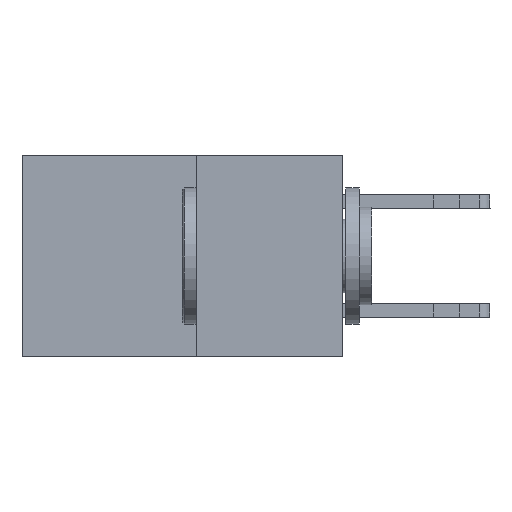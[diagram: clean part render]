
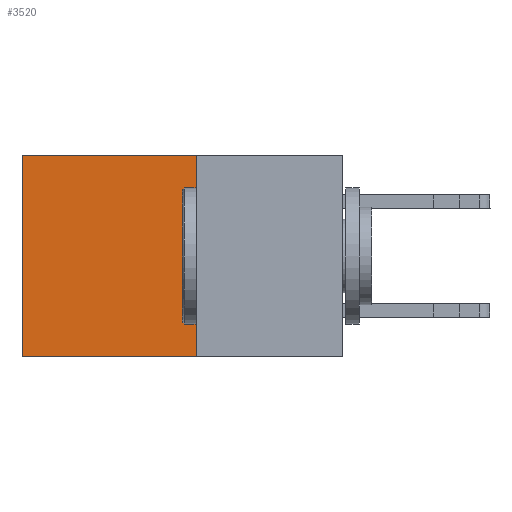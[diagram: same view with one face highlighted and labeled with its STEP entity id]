
A CAD part, left-side view. The second image highlights one B-rep face of the part: STEP entity #3520.
In plain terms, the highlighted planar face has unit normal (-1, 0, 0).
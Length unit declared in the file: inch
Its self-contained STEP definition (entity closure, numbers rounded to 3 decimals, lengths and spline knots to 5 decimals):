
#206 = VECTOR ( 'NONE', #11666, 39.37008 ) ;
#551 = VECTOR ( 'NONE', #7633, 39.37008 ) ;
#1051 = CARTESIAN_POINT ( 'NONE',  ( 0.277, 0.27, -0.37 ) ) ;
#2357 = EDGE_CURVE ( 'NONE', #12466, #11391, #11826, .T. ) ;
#2805 = LINE ( 'NONE', #3881, #5023 ) ;
#3520 = ADVANCED_FACE ( 'NONE', ( #3903 ), #9581, .F. ) ;
#3819 = EDGE_CURVE ( 'NONE', #10381, #12466, #8734, .T. ) ;
#3881 = CARTESIAN_POINT ( 'NONE',  ( 0.277, 0.27, -0.37 ) ) ;
#3903 = FACE_OUTER_BOUND ( 'NONE', #8904, .T. ) ;
#4460 = ORIENTED_EDGE ( 'NONE', *, *, #7436, .F. ) ;
#4825 = ORIENTED_EDGE ( 'NONE', *, *, #9053, .F. ) ;
#4991 = DIRECTION ( 'NONE',  ( 0., 0., -1. ) ) ;
#5023 = VECTOR ( 'NONE', #4991, 39.37008 ) ;
#5216 = CARTESIAN_POINT ( 'NONE',  ( 0.277, 0.59, 0. ) ) ;
#5542 = LINE ( 'NONE', #1051, #7706 ) ;
#5982 = DIRECTION ( 'NONE',  ( 0., 0., -1. ) ) ;
#6345 = DIRECTION ( 'NONE',  ( 1., 0., 0. ) ) ;
#7020 = CARTESIAN_POINT ( 'NONE',  ( 0.277, 0.27, 0. ) ) ;
#7436 = EDGE_CURVE ( 'NONE', #13452, #11391, #5542, .T. ) ;
#7629 = ORIENTED_EDGE ( 'NONE', *, *, #3819, .T. ) ;
#7633 = DIRECTION ( 'NONE',  ( 0., 0., -1. ) ) ;
#7706 = VECTOR ( 'NONE', #10640, 39.37008 ) ;
#7736 = CARTESIAN_POINT ( 'NONE',  ( 0.277, 0.59, -0.37 ) ) ;
#8416 = CARTESIAN_POINT ( 'NONE',  ( 0.277, 0.27, -0.37 ) ) ;
#8734 = LINE ( 'NONE', #12720, #206 ) ;
#8800 = CARTESIAN_POINT ( 'NONE',  ( 0.277, 0.59, -0.37 ) ) ;
#8904 = EDGE_LOOP ( 'NONE', ( #9752, #4460, #4825, #7629 ) ) ;
#9053 = EDGE_CURVE ( 'NONE', #10381, #13452, #2805, .T. ) ;
#9581 = PLANE ( 'NONE',  #11363 ) ;
#9752 = ORIENTED_EDGE ( 'NONE', *, *, #2357, .T. ) ;
#10381 = VERTEX_POINT ( 'NONE', #7020 ) ;
#10597 = CARTESIAN_POINT ( 'NONE',  ( 0.277, 0.27, -0.37 ) ) ;
#10640 = DIRECTION ( 'NONE',  ( 0., 1., 0. ) ) ;
#11363 = AXIS2_PLACEMENT_3D ( 'NONE', #10597, #6345, #5982 ) ;
#11391 = VERTEX_POINT ( 'NONE', #7736 ) ;
#11666 = DIRECTION ( 'NONE',  ( 0., 1., 0. ) ) ;
#11826 = LINE ( 'NONE', #8800, #551 ) ;
#12466 = VERTEX_POINT ( 'NONE', #5216 ) ;
#12720 = CARTESIAN_POINT ( 'NONE',  ( 0.277, 0.27, 0. ) ) ;
#13452 = VERTEX_POINT ( 'NONE', #8416 ) ;
